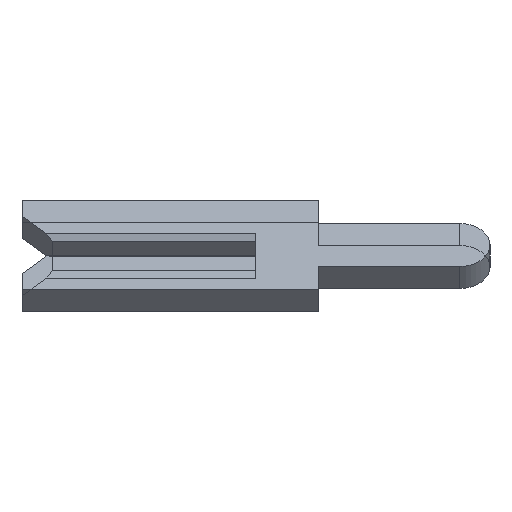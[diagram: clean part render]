
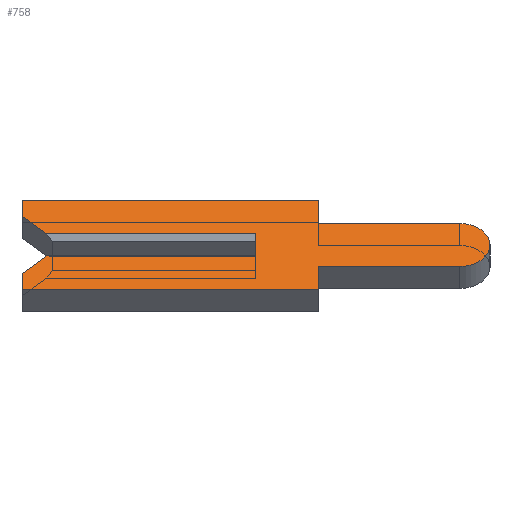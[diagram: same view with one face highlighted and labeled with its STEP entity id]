
A CAD part, left-side view. The second image highlights one B-rep face of the part: STEP entity #758.
In plain terms, the highlighted face is planar.
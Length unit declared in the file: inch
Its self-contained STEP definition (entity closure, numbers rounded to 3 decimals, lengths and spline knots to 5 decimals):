
#9 = VERTEX_POINT ( 'NONE', #2223 ) ;
#25 = VERTEX_POINT ( 'NONE', #572 ) ;
#54 = ORIENTED_EDGE ( 'NONE', *, *, #1418, .F. ) ;
#78 = CARTESIAN_POINT ( 'NONE',  ( -0.01, -0.04, 0.04 ) ) ;
#105 = ORIENTED_EDGE ( 'NONE', *, *, #813, .F. ) ;
#152 = CARTESIAN_POINT ( 'NONE',  ( -0.01, -0.1305, -0.01 ) ) ;
#177 = VECTOR ( 'NONE', #375, 39.37008 ) ;
#189 = CARTESIAN_POINT ( 'NONE',  ( -0.01, -0.04, 0.04 ) ) ;
#191 = CARTESIAN_POINT ( 'NONE',  ( -0.01, 0., -0.01 ) ) ;
#192 = EDGE_CURVE ( 'NONE', #1280, #1959, #408, .T. ) ;
#228 = LINE ( 'NONE', #1752, #350 ) ;
#244 = CIRCLE ( 'NONE', #2219, 0.0195 ) ;
#257 = VERTEX_POINT ( 'NONE', #741 ) ;
#266 = VERTEX_POINT ( 'NONE', #191 ) ;
#268 = CARTESIAN_POINT ( 'NONE',  ( -0.01, -0.1305, 0. ) ) ;
#324 = EDGE_CURVE ( 'NONE', #2019, #9, #634, .T. ) ;
#334 = DIRECTION ( 'NONE',  ( 0., -1., 0. ) ) ;
#350 = VECTOR ( 'NONE', #1713, 39.37008 ) ;
#375 = DIRECTION ( 'NONE',  ( 0., -0.707, 0.707 ) ) ;
#384 = ORIENTED_EDGE ( 'NONE', *, *, #1952, .F. ) ;
#408 = LINE ( 'NONE', #2242, #1221 ) ;
#476 = VECTOR ( 'NONE', #334, 39.37008 ) ;
#492 = EDGE_CURVE ( 'NONE', #257, #1280, #228, .T. ) ;
#533 = FACE_OUTER_BOUND ( 'NONE', #677, .T. ) ;
#540 = CARTESIAN_POINT ( 'NONE',  ( -0.01, 0.15, -0.026 ) ) ;
#554 = LINE ( 'NONE', #1014, #791 ) ;
#568 = ORIENTED_EDGE ( 'NONE', *, *, #1750, .F. ) ;
#572 = CARTESIAN_POINT ( 'NONE',  ( -0.01, 0.15, 0.026 ) ) ;
#589 = ORIENTED_EDGE ( 'NONE', *, *, #1657, .F. ) ;
#626 = DIRECTION ( 'NONE',  ( 0., 0., -1. ) ) ;
#634 = LINE ( 'NONE', #809, #747 ) ;
#647 = VECTOR ( 'NONE', #1993, 39.37008 ) ;
#664 = CARTESIAN_POINT ( 'NONE',  ( -0.01, -0.04, -0.04 ) ) ;
#677 = EDGE_LOOP ( 'NONE', ( #1520, #1937, #568, #54, #384, #2271, #1376, #1135, #589, #1866, #1548, #1394, #832, #105 ) ) ;
#687 = CARTESIAN_POINT ( 'NONE',  ( -0.01, 0., 0.0065 ) ) ;
#700 = LINE ( 'NONE', #687, #647 ) ;
#727 = EDGE_CURVE ( 'NONE', #2360, #2019, #1643, .T. ) ;
#741 = CARTESIAN_POINT ( 'NONE',  ( -0.01, -0.04, -0.0195 ) ) ;
#747 = VECTOR ( 'NONE', #2103, 39.37008 ) ;
#758 = ADVANCED_FACE ( 'NONE', ( #533 ), #1379, .F. ) ;
#764 = CARTESIAN_POINT ( 'NONE',  ( -0.01, -0.04, 0.0195 ) ) ;
#787 = EDGE_CURVE ( 'NONE', #1501, #257, #554, .T. ) ;
#791 = VECTOR ( 'NONE', #2344, 39.37008 ) ;
#809 = CARTESIAN_POINT ( 'NONE',  ( -0.01, -0.04, 0.0195 ) ) ;
#813 = EDGE_CURVE ( 'NONE', #1270, #25, #1797, .T. ) ;
#832 = ORIENTED_EDGE ( 'NONE', *, *, #1711, .F. ) ;
#862 = CARTESIAN_POINT ( 'NONE',  ( -0.01, 0.15, 0.04 ) ) ;
#875 = LINE ( 'NONE', #152, #1144 ) ;
#899 = CARTESIAN_POINT ( 'NONE',  ( -0.01, 0.1305, -0.0065 ) ) ;
#903 = LINE ( 'NONE', #1710, #1076 ) ;
#918 = CARTESIAN_POINT ( 'NONE',  ( -0.01, -0.1305, -0.0195 ) ) ;
#967 = LINE ( 'NONE', #862, #476 ) ;
#988 = EDGE_CURVE ( 'NONE', #266, #2153, #700, .T. ) ;
#998 = DIRECTION ( 'NONE',  ( 0., 0.707, 0.707 ) ) ;
#1014 = CARTESIAN_POINT ( 'NONE',  ( -0.01, -0.04, -0.0195 ) ) ;
#1069 = EDGE_CURVE ( 'NONE', #1270, #2153, #2086, .T. ) ;
#1076 = VECTOR ( 'NONE', #1693, 39.37008 ) ;
#1077 = DIRECTION ( 'NONE',  ( 1., 0., 0. ) ) ;
#1080 = VECTOR ( 'NONE', #2155, 39.37008 ) ;
#1100 = DIRECTION ( 'NONE',  ( 0., 0., 1. ) ) ;
#1128 = CARTESIAN_POINT ( 'NONE',  ( -0.01, 0., 0.01 ) ) ;
#1135 = ORIENTED_EDGE ( 'NONE', *, *, #787, .F. ) ;
#1144 = VECTOR ( 'NONE', #1639, 39.37008 ) ;
#1198 = VERTEX_POINT ( 'NONE', #1244 ) ;
#1213 = DIRECTION ( 'NONE',  ( 1., 0., 0. ) ) ;
#1220 = EDGE_CURVE ( 'NONE', #2092, #2360, #967, .T. ) ;
#1221 = VECTOR ( 'NONE', #1487, 39.37008 ) ;
#1244 = CARTESIAN_POINT ( 'NONE',  ( -0.01, 0.134, -0.01 ) ) ;
#1262 = AXIS2_PLACEMENT_3D ( 'NONE', #268, #1213, #626 ) ;
#1270 = VERTEX_POINT ( 'NONE', #2175 ) ;
#1280 = VERTEX_POINT ( 'NONE', #664 ) ;
#1317 = CARTESIAN_POINT ( 'NONE',  ( -0.01, 0.15, 0.04 ) ) ;
#1376 = ORIENTED_EDGE ( 'NONE', *, *, #492, .F. ) ;
#1379 = PLANE ( 'NONE',  #1262 ) ;
#1394 = ORIENTED_EDGE ( 'NONE', *, *, #1220, .F. ) ;
#1417 = VECTOR ( 'NONE', #998, 39.37008 ) ;
#1418 = EDGE_CURVE ( 'NONE', #1484, #1198, #2352, .T. ) ;
#1484 = VERTEX_POINT ( 'NONE', #540 ) ;
#1487 = DIRECTION ( 'NONE',  ( 0., 1., 0. ) ) ;
#1501 = VERTEX_POINT ( 'NONE', #918 ) ;
#1520 = ORIENTED_EDGE ( 'NONE', *, *, #1069, .T. ) ;
#1548 = ORIENTED_EDGE ( 'NONE', *, *, #727, .F. ) ;
#1582 = VECTOR ( 'NONE', #1100, 39.37008 ) ;
#1639 = DIRECTION ( 'NONE',  ( 0., -1., 0. ) ) ;
#1643 = LINE ( 'NONE', #78, #2166 ) ;
#1652 = CARTESIAN_POINT ( 'NONE',  ( -0.01, 0.15, 0.026 ) ) ;
#1657 = EDGE_CURVE ( 'NONE', #9, #1501, #244, .T. ) ;
#1693 = DIRECTION ( 'NONE',  ( 0., 0., 1. ) ) ;
#1710 = CARTESIAN_POINT ( 'NONE',  ( -0.01, 0.15, -0.026 ) ) ;
#1711 = EDGE_CURVE ( 'NONE', #25, #2092, #2162, .T. ) ;
#1713 = DIRECTION ( 'NONE',  ( 0., 0., -1. ) ) ;
#1717 = CARTESIAN_POINT ( 'NONE',  ( -0.01, 0.15, -0.04 ) ) ;
#1750 = EDGE_CURVE ( 'NONE', #1198, #266, #875, .T. ) ;
#1752 = CARTESIAN_POINT ( 'NONE',  ( -0.01, -0.04, -0.04 ) ) ;
#1781 = CARTESIAN_POINT ( 'NONE',  ( -0.01, 0.1305, 0.0065 ) ) ;
#1797 = LINE ( 'NONE', #1781, #1417 ) ;
#1820 = CARTESIAN_POINT ( 'NONE',  ( -0.01, 0.15, 0.01 ) ) ;
#1866 = ORIENTED_EDGE ( 'NONE', *, *, #324, .F. ) ;
#1937 = ORIENTED_EDGE ( 'NONE', *, *, #988, .F. ) ;
#1952 = EDGE_CURVE ( 'NONE', #1959, #1484, #903, .T. ) ;
#1959 = VERTEX_POINT ( 'NONE', #1717 ) ;
#1993 = DIRECTION ( 'NONE',  ( 0., 0., 1. ) ) ;
#2019 = VERTEX_POINT ( 'NONE', #764 ) ;
#2041 = DIRECTION ( 'NONE',  ( 0., 0., -1. ) ) ;
#2086 = LINE ( 'NONE', #1820, #1080 ) ;
#2092 = VERTEX_POINT ( 'NONE', #1317 ) ;
#2103 = DIRECTION ( 'NONE',  ( 0., -1., 0. ) ) ;
#2153 = VERTEX_POINT ( 'NONE', #1128 ) ;
#2155 = DIRECTION ( 'NONE',  ( 0., -1., 0. ) ) ;
#2162 = LINE ( 'NONE', #1652, #1582 ) ;
#2166 = VECTOR ( 'NONE', #2339, 39.37008 ) ;
#2175 = CARTESIAN_POINT ( 'NONE',  ( -0.01, 0.134, 0.01 ) ) ;
#2219 = AXIS2_PLACEMENT_3D ( 'NONE', #2237, #1077, #2041 ) ;
#2223 = CARTESIAN_POINT ( 'NONE',  ( -0.01, -0.1305, 0.0195 ) ) ;
#2237 = CARTESIAN_POINT ( 'NONE',  ( -0.01, -0.1305, 0. ) ) ;
#2242 = CARTESIAN_POINT ( 'NONE',  ( -0.01, 0.15, -0.04 ) ) ;
#2271 = ORIENTED_EDGE ( 'NONE', *, *, #192, .F. ) ;
#2339 = DIRECTION ( 'NONE',  ( 0., 0., -1. ) ) ;
#2344 = DIRECTION ( 'NONE',  ( 0., 1., 0. ) ) ;
#2352 = LINE ( 'NONE', #899, #177 ) ;
#2360 = VERTEX_POINT ( 'NONE', #189 ) ;
